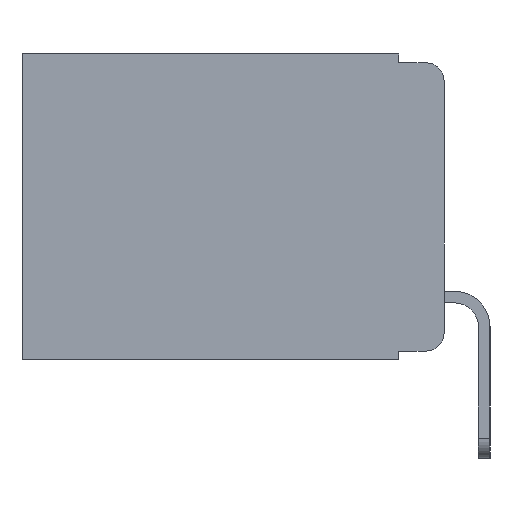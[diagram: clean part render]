
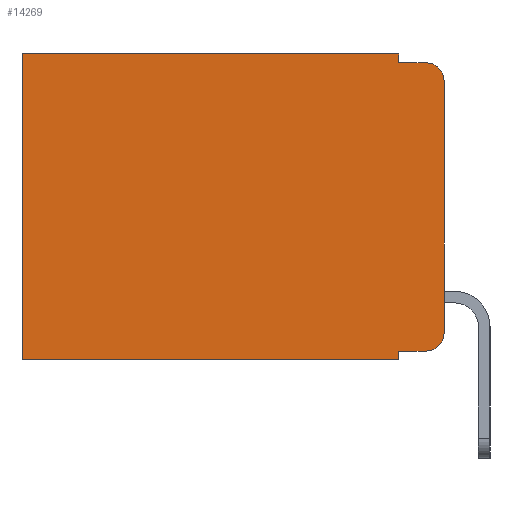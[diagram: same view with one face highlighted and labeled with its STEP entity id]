
A CAD part, left-side view. The second image highlights one B-rep face of the part: STEP entity #14269.
In plain terms, the highlighted planar face has unit normal (-1, 0, 0).
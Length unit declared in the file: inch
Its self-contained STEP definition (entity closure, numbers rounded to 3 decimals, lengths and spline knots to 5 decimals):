
#347 = VERTEX_POINT ( 'NONE', #9037 ) ;
#681 = EDGE_CURVE ( 'NONE', #17011, #9704, #2575, .T. ) ;
#1557 = EDGE_CURVE ( 'NONE', #15442, #3338, #6018, .T. ) ;
#1921 = VECTOR ( 'NONE', #8534, 39.37008 ) ;
#1970 = PLANE ( 'NONE',  #13211 ) ;
#2095 = EDGE_CURVE ( 'NONE', #13973, #347, #19518, .T. ) ;
#2138 = EDGE_CURVE ( 'NONE', #13973, #14397, #13479, .T. ) ;
#2224 = EDGE_CURVE ( 'NONE', #11848, #14397, #11928, .T. ) ;
#2262 = EDGE_CURVE ( 'NONE', #17011, #11848, #3096, .T. ) ;
#2267 = EDGE_CURVE ( 'NONE', #9704, #3338, #15291, .T. ) ;
#2298 = DIRECTION ( 'NONE',  ( 0., 0., -1. ) ) ;
#2302 = EDGE_CURVE ( 'NONE', #3480, #15442, #6021, .T. ) ;
#2329 = EDGE_CURVE ( 'NONE', #3480, #7990, #18404, .T. ) ;
#2336 = EDGE_CURVE ( 'NONE', #7990, #347, #5039, .T. ) ;
#2575 = LINE ( 'NONE', #18079, #15326 ) ;
#2859 = ORIENTED_EDGE ( 'NONE', *, *, #1557, .F. ) ;
#3096 = LINE ( 'NONE', #3993, #15795 ) ;
#3338 = VERTEX_POINT ( 'NONE', #9336 ) ;
#3480 = VERTEX_POINT ( 'NONE', #8757 ) ;
#3993 = CARTESIAN_POINT ( 'NONE',  ( 0.298, 0.051, 0. ) ) ;
#4566 = CARTESIAN_POINT ( 'NONE',  ( 0.298, 0.051, -0.343 ) ) ;
#5039 = CIRCLE ( 'NONE', #16786, 0.02 ) ;
#5062 = CARTESIAN_POINT ( 'NONE',  ( 0.298, 0., -0.343 ) ) ;
#5205 = CARTESIAN_POINT ( 'NONE',  ( 0.298, 0.051, 0. ) ) ;
#5397 = DIRECTION ( 'NONE',  ( 0., 0., -1. ) ) ;
#5573 = CARTESIAN_POINT ( 'NONE',  ( 0.298, 0., 0. ) ) ;
#6018 = LINE ( 'NONE', #5062, #14228 ) ;
#6021 = LINE ( 'NONE', #5205, #9855 ) ;
#6296 = ORIENTED_EDGE ( 'NONE', *, *, #2302, .F. ) ;
#6564 = DIRECTION ( 'NONE',  ( 0., -1., 0. ) ) ;
#6710 = CARTESIAN_POINT ( 'NONE',  ( 0.298, 0.051, -0.01 ) ) ;
#7129 = DIRECTION ( 'NONE',  ( 0., 0., -1. ) ) ;
#7314 = ORIENTED_EDGE ( 'NONE', *, *, #2329, .T. ) ;
#7522 = CARTESIAN_POINT ( 'NONE',  ( 0.298, 0.02, -0.313 ) ) ;
#7884 = CARTESIAN_POINT ( 'NONE',  ( 0.298, 0., 0. ) ) ;
#7943 = ORIENTED_EDGE ( 'NONE', *, *, #2336, .T. ) ;
#7948 = AXIS2_PLACEMENT_3D ( 'NONE', #16101, #16081, #15951 ) ;
#7990 = VERTEX_POINT ( 'NONE', #11604 ) ;
#8534 = DIRECTION ( 'NONE',  ( 0., 0., -1. ) ) ;
#8757 = CARTESIAN_POINT ( 'NONE',  ( 0.298, 0.051, -0.333 ) ) ;
#9037 = CARTESIAN_POINT ( 'NONE',  ( 0.298, 0., -0.313 ) ) ;
#9056 = DIRECTION ( 'NONE',  ( 0., 0., -1. ) ) ;
#9336 = CARTESIAN_POINT ( 'NONE',  ( 0.298, 0.473, -0.343 ) ) ;
#9704 = VERTEX_POINT ( 'NONE', #19512 ) ;
#9855 = VECTOR ( 'NONE', #9056, 39.37008 ) ;
#10916 = DIRECTION ( 'NONE',  ( 0., 1., 0. ) ) ;
#11321 = CARTESIAN_POINT ( 'NONE',  ( 0.298, 0., -0.03 ) ) ;
#11604 = CARTESIAN_POINT ( 'NONE',  ( 0.298, 0.02, -0.333 ) ) ;
#11848 = VERTEX_POINT ( 'NONE', #14611 ) ;
#11928 = LINE ( 'NONE', #6710, #19735 ) ;
#13112 = FACE_OUTER_BOUND ( 'NONE', #13557, .T. ) ;
#13211 = AXIS2_PLACEMENT_3D ( 'NONE', #5573, #16940, #7129 ) ;
#13479 = CIRCLE ( 'NONE', #7948, 0.02 ) ;
#13557 = EDGE_LOOP ( 'NONE', ( #15517, #16641, #17758, #18568, #19822, #14729, #2859, #6296, #7314, #7943 ) ) ;
#13670 = CARTESIAN_POINT ( 'NONE',  ( 0.298, 0.051, 0. ) ) ;
#13973 = VERTEX_POINT ( 'NONE', #11321 ) ;
#14108 = CARTESIAN_POINT ( 'NONE',  ( 0.298, 0.02, -0.01 ) ) ;
#14228 = VECTOR ( 'NONE', #17379, 39.37008 ) ;
#14269 = ADVANCED_FACE ( 'NONE', ( #13112 ), #1970, .F. ) ;
#14397 = VERTEX_POINT ( 'NONE', #14108 ) ;
#14490 = VECTOR ( 'NONE', #5397, 39.37008 ) ;
#14611 = CARTESIAN_POINT ( 'NONE',  ( 0.298, 0.051, -0.01 ) ) ;
#14624 = CARTESIAN_POINT ( 'NONE',  ( 0.298, 0.051, -0.333 ) ) ;
#14729 = ORIENTED_EDGE ( 'NONE', *, *, #2267, .T. ) ;
#15291 = LINE ( 'NONE', #18962, #1921 ) ;
#15326 = VECTOR ( 'NONE', #10916, 39.37008 ) ;
#15442 = VERTEX_POINT ( 'NONE', #4566 ) ;
#15517 = ORIENTED_EDGE ( 'NONE', *, *, #2095, .F. ) ;
#15795 = VECTOR ( 'NONE', #2298, 39.37008 ) ;
#15951 = DIRECTION ( 'NONE',  ( 0., 0., -1. ) ) ;
#16081 = DIRECTION ( 'NONE',  ( -1., 0., 0. ) ) ;
#16101 = CARTESIAN_POINT ( 'NONE',  ( 0.298, 0.02, -0.03 ) ) ;
#16641 = ORIENTED_EDGE ( 'NONE', *, *, #2138, .T. ) ;
#16786 = AXIS2_PLACEMENT_3D ( 'NONE', #7522, #18049, #20980 ) ;
#16940 = DIRECTION ( 'NONE',  ( 1., 0., 0. ) ) ;
#17011 = VERTEX_POINT ( 'NONE', #13670 ) ;
#17379 = DIRECTION ( 'NONE',  ( 0., 1., 0. ) ) ;
#17758 = ORIENTED_EDGE ( 'NONE', *, *, #2224, .F. ) ;
#17952 = VECTOR ( 'NONE', #20652, 39.37008 ) ;
#18049 = DIRECTION ( 'NONE',  ( -1., 0., 0. ) ) ;
#18079 = CARTESIAN_POINT ( 'NONE',  ( 0.298, 0., 0. ) ) ;
#18404 = LINE ( 'NONE', #14624, #17952 ) ;
#18568 = ORIENTED_EDGE ( 'NONE', *, *, #2262, .F. ) ;
#18962 = CARTESIAN_POINT ( 'NONE',  ( 0.298, 0.473, 0. ) ) ;
#19512 = CARTESIAN_POINT ( 'NONE',  ( 0.298, 0.473, 0. ) ) ;
#19518 = LINE ( 'NONE', #7884, #14490 ) ;
#19735 = VECTOR ( 'NONE', #6564, 39.37008 ) ;
#19822 = ORIENTED_EDGE ( 'NONE', *, *, #681, .T. ) ;
#20652 = DIRECTION ( 'NONE',  ( 0., -1., 0. ) ) ;
#20980 = DIRECTION ( 'NONE',  ( 0., 0., -1. ) ) ;
